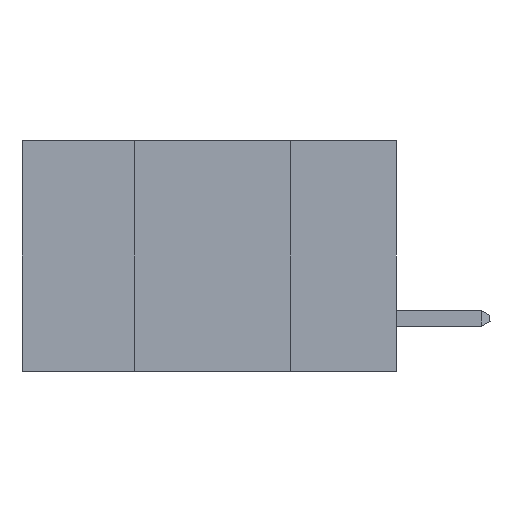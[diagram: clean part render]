
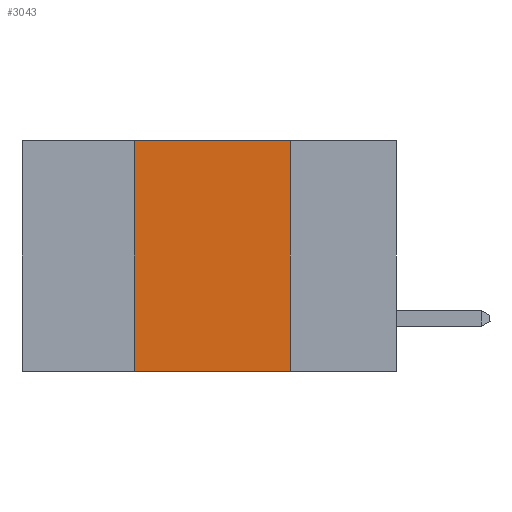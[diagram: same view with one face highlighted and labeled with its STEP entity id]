
A CAD part, left-side view. The second image highlights one B-rep face of the part: STEP entity #3043.
In plain terms, the highlighted planar face has unit normal (-1, 0, 0).
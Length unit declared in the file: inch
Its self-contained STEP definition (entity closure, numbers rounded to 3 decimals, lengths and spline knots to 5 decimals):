
#1973 = LINE ( 'NONE', #4476, #6937 ) ;
#3043 = ADVANCED_FACE ( 'NONE', ( #7196 ), #11823, .F. ) ;
#3711 = CARTESIAN_POINT ( 'NONE',  ( 0., 0.42, 0. ) ) ;
#3830 = EDGE_CURVE ( 'NONE', #19185, #19291, #15623, .T. ) ;
#4191 = VECTOR ( 'NONE', #13929, 39.37008 ) ;
#4476 = CARTESIAN_POINT ( 'NONE',  ( 0., 0.6, 0. ) ) ;
#4557 = VECTOR ( 'NONE', #6775, 39.37008 ) ;
#5000 = CARTESIAN_POINT ( 'NONE',  ( 0., 0.17, -0.37 ) ) ;
#5055 = VECTOR ( 'NONE', #18955, 39.37008 ) ;
#5069 = EDGE_CURVE ( 'NONE', #21451, #10769, #10041, .T. ) ;
#5736 = ORIENTED_EDGE ( 'NONE', *, *, #3830, .F. ) ;
#6753 = CARTESIAN_POINT ( 'NONE',  ( 0., 0.42, -0.37 ) ) ;
#6775 = DIRECTION ( 'NONE',  ( 0., 0., 1. ) ) ;
#6875 = CARTESIAN_POINT ( 'NONE',  ( 0., 0.17, 0. ) ) ;
#6937 = VECTOR ( 'NONE', #15635, 39.37008 ) ;
#7196 = FACE_OUTER_BOUND ( 'NONE', #14810, .T. ) ;
#9024 = CARTESIAN_POINT ( 'NONE',  ( 0., 0.42, 0. ) ) ;
#9138 = LINE ( 'NONE', #17524, #4191 ) ;
#10041 = LINE ( 'NONE', #20585, #5055 ) ;
#10583 = EDGE_CURVE ( 'NONE', #19185, #10769, #9138, .T. ) ;
#10769 = VERTEX_POINT ( 'NONE', #5000 ) ;
#11777 = DIRECTION ( 'NONE',  ( 1., 0., 0. ) ) ;
#11823 = PLANE ( 'NONE',  #19861 ) ;
#13258 = DIRECTION ( 'NONE',  ( 0., 0., -1. ) ) ;
#13864 = ORIENTED_EDGE ( 'NONE', *, *, #10583, .T. ) ;
#13929 = DIRECTION ( 'NONE',  ( 0., -1., 0. ) ) ;
#14810 = EDGE_LOOP ( 'NONE', ( #20463, #17114, #5736, #13864 ) ) ;
#15623 = LINE ( 'NONE', #3711, #4557 ) ;
#15635 = DIRECTION ( 'NONE',  ( 0., -1., 0. ) ) ;
#17114 = ORIENTED_EDGE ( 'NONE', *, *, #22476, .F. ) ;
#17524 = CARTESIAN_POINT ( 'NONE',  ( 0., 0.6, -0.37 ) ) ;
#18955 = DIRECTION ( 'NONE',  ( 0., 0., -1. ) ) ;
#19185 = VERTEX_POINT ( 'NONE', #6753 ) ;
#19291 = VERTEX_POINT ( 'NONE', #9024 ) ;
#19861 = AXIS2_PLACEMENT_3D ( 'NONE', #23007, #11777, #13258 ) ;
#20463 = ORIENTED_EDGE ( 'NONE', *, *, #5069, .F. ) ;
#20585 = CARTESIAN_POINT ( 'NONE',  ( 0., 0.17, 0. ) ) ;
#21451 = VERTEX_POINT ( 'NONE', #6875 ) ;
#22476 = EDGE_CURVE ( 'NONE', #19291, #21451, #1973, .T. ) ;
#23007 = CARTESIAN_POINT ( 'NONE',  ( 0., 0.6, 0. ) ) ;
